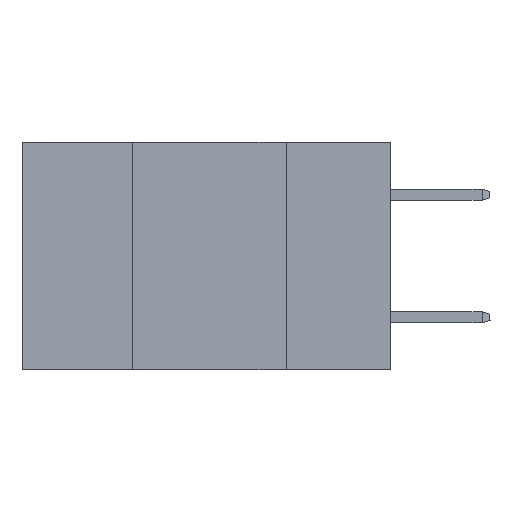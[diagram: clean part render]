
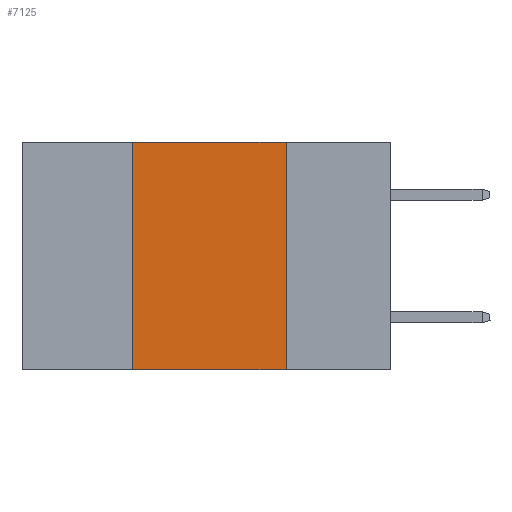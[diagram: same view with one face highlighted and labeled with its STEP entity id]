
A CAD part, left-side view. The second image highlights one B-rep face of the part: STEP entity #7125.
In plain terms, the highlighted planar face has unit normal (-1, 0, 0).
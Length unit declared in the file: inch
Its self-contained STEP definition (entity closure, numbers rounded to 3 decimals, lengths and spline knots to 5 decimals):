
#1175 = LINE ( 'NONE', #5291, #19985 ) ;
#1581 = CARTESIAN_POINT ( 'NONE',  ( 0., 0.6, 0. ) ) ;
#1677 = CARTESIAN_POINT ( 'NONE',  ( 0., 0.17, 0. ) ) ;
#2044 = VERTEX_POINT ( 'NONE', #13515 ) ;
#2268 = CARTESIAN_POINT ( 'NONE',  ( 0., 0.42, -0.37 ) ) ;
#4316 = EDGE_CURVE ( 'NONE', #22301, #17984, #17902, .T. ) ;
#5001 = VECTOR ( 'NONE', #7690, 39.37008 ) ;
#5291 = CARTESIAN_POINT ( 'NONE',  ( 0., 0.6, 0. ) ) ;
#5848 = DIRECTION ( 'NONE',  ( 0., 0., -1. ) ) ;
#5967 = DIRECTION ( 'NONE',  ( 1., 0., 0. ) ) ;
#6575 = CARTESIAN_POINT ( 'NONE',  ( 0., 0.17, -0.37 ) ) ;
#6629 = LINE ( 'NONE', #15460, #15732 ) ;
#6639 = EDGE_LOOP ( 'NONE', ( #25377, #24107, #13084, #19847 ) ) ;
#7125 = ADVANCED_FACE ( 'NONE', ( #24631 ), #24231, .F. ) ;
#7690 = DIRECTION ( 'NONE',  ( 0., 0., -1. ) ) ;
#11958 = VECTOR ( 'NONE', #15228, 39.37008 ) ;
#13084 = ORIENTED_EDGE ( 'NONE', *, *, #4316, .F. ) ;
#13515 = CARTESIAN_POINT ( 'NONE',  ( 0., 0.17, 0. ) ) ;
#13982 = EDGE_CURVE ( 'NONE', #2044, #14561, #21562, .T. ) ;
#14240 = AXIS2_PLACEMENT_3D ( 'NONE', #1581, #5967, #5848 ) ;
#14561 = VERTEX_POINT ( 'NONE', #6575 ) ;
#15228 = DIRECTION ( 'NONE',  ( 0., 0., 1. ) ) ;
#15460 = CARTESIAN_POINT ( 'NONE',  ( 0., 0.6, -0.37 ) ) ;
#15732 = VECTOR ( 'NONE', #25012, 39.37008 ) ;
#16914 = EDGE_CURVE ( 'NONE', #17984, #2044, #1175, .T. ) ;
#17902 = LINE ( 'NONE', #19647, #11958 ) ;
#17984 = VERTEX_POINT ( 'NONE', #20566 ) ;
#19452 = EDGE_CURVE ( 'NONE', #22301, #14561, #6629, .T. ) ;
#19647 = CARTESIAN_POINT ( 'NONE',  ( 0., 0.42, 0. ) ) ;
#19847 = ORIENTED_EDGE ( 'NONE', *, *, #19452, .T. ) ;
#19985 = VECTOR ( 'NONE', #25816, 39.37008 ) ;
#20566 = CARTESIAN_POINT ( 'NONE',  ( 0., 0.42, 0. ) ) ;
#21562 = LINE ( 'NONE', #1677, #5001 ) ;
#22301 = VERTEX_POINT ( 'NONE', #2268 ) ;
#24107 = ORIENTED_EDGE ( 'NONE', *, *, #16914, .F. ) ;
#24231 = PLANE ( 'NONE',  #14240 ) ;
#24631 = FACE_OUTER_BOUND ( 'NONE', #6639, .T. ) ;
#25012 = DIRECTION ( 'NONE',  ( 0., -1., 0. ) ) ;
#25377 = ORIENTED_EDGE ( 'NONE', *, *, #13982, .F. ) ;
#25816 = DIRECTION ( 'NONE',  ( 0., -1., 0. ) ) ;
